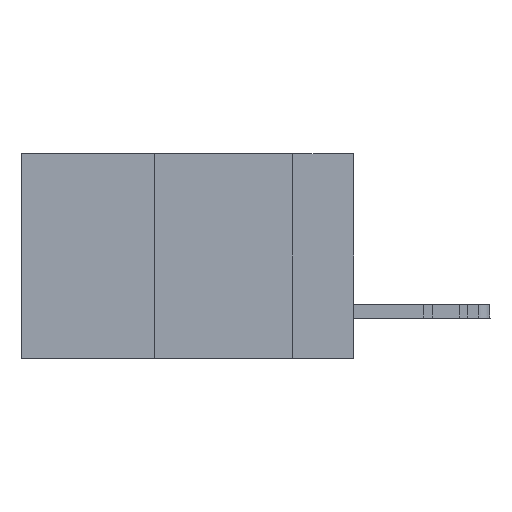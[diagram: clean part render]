
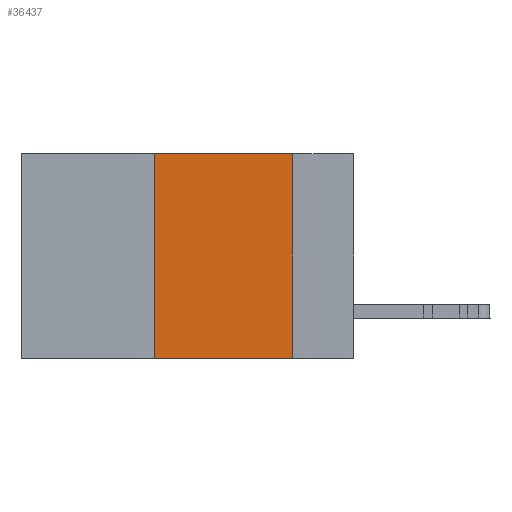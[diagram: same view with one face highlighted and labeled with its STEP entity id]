
A CAD part, left-side view. The second image highlights one B-rep face of the part: STEP entity #36437.
In plain terms, the highlighted planar face has unit normal (-1, 0, 0).
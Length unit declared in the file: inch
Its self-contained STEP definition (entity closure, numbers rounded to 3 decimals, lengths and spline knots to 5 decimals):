
#14 = LINE ( 'NONE', #45840, #43859 ) ;
#899 = ORIENTED_EDGE ( 'NONE', *, *, #42358, .F. ) ;
#2117 = DIRECTION ( 'NONE',  ( 0., 0., -1. ) ) ;
#2658 = VERTEX_POINT ( 'NONE', #26559 ) ;
#3344 = LINE ( 'NONE', #26875, #9012 ) ;
#9012 = VECTOR ( 'NONE', #49640, 39.37008 ) ;
#11147 = LINE ( 'NONE', #22791, #41113 ) ;
#11710 = ORIENTED_EDGE ( 'NONE', *, *, #39210, .F. ) ;
#12182 = DIRECTION ( 'NONE',  ( 0., 0., -1. ) ) ;
#12273 = VERTEX_POINT ( 'NONE', #48362 ) ;
#13768 = DIRECTION ( 'NONE',  ( 1., 0., 0. ) ) ;
#14005 = CARTESIAN_POINT ( 'NONE',  ( 0., 0.36, 0. ) ) ;
#16479 = CARTESIAN_POINT ( 'NONE',  ( 0., 0.11, -0.37 ) ) ;
#17064 = EDGE_CURVE ( 'NONE', #33422, #12273, #11147, .T. ) ;
#20358 = ORIENTED_EDGE ( 'NONE', *, *, #17064, .F. ) ;
#21111 = PLANE ( 'NONE',  #38744 ) ;
#22791 = CARTESIAN_POINT ( 'NONE',  ( 0., 0.6, 0. ) ) ;
#24957 = ORIENTED_EDGE ( 'NONE', *, *, #36163, .T. ) ;
#26559 = CARTESIAN_POINT ( 'NONE',  ( 0., 0.36, -0.37 ) ) ;
#26875 = CARTESIAN_POINT ( 'NONE',  ( 0., 0.36, 0. ) ) ;
#33422 = VERTEX_POINT ( 'NONE', #14005 ) ;
#34288 = CARTESIAN_POINT ( 'NONE',  ( 0., 0.6, -0.37 ) ) ;
#34822 = EDGE_LOOP ( 'NONE', ( #899, #20358, #11710, #24957 ) ) ;
#36163 = EDGE_CURVE ( 'NONE', #2658, #49295, #37347, .T. ) ;
#36437 = ADVANCED_FACE ( 'NONE', ( #39847 ), #21111, .F. ) ;
#37347 = LINE ( 'NONE', #34288, #45164 ) ;
#38230 = DIRECTION ( 'NONE',  ( 0., -1., 0. ) ) ;
#38744 = AXIS2_PLACEMENT_3D ( 'NONE', #40333, #13768, #2117 ) ;
#39210 = EDGE_CURVE ( 'NONE', #2658, #33422, #3344, .T. ) ;
#39847 = FACE_OUTER_BOUND ( 'NONE', #34822, .T. ) ;
#40333 = CARTESIAN_POINT ( 'NONE',  ( 0., 0.6, 0. ) ) ;
#41113 = VECTOR ( 'NONE', #38230, 39.37008 ) ;
#42358 = EDGE_CURVE ( 'NONE', #12273, #49295, #14, .T. ) ;
#43859 = VECTOR ( 'NONE', #12182, 39.37008 ) ;
#45164 = VECTOR ( 'NONE', #46178, 39.37008 ) ;
#45840 = CARTESIAN_POINT ( 'NONE',  ( 0., 0.11, 0. ) ) ;
#46178 = DIRECTION ( 'NONE',  ( 0., -1., 0. ) ) ;
#48362 = CARTESIAN_POINT ( 'NONE',  ( 0., 0.11, 0. ) ) ;
#49295 = VERTEX_POINT ( 'NONE', #16479 ) ;
#49640 = DIRECTION ( 'NONE',  ( 0., 0., 1. ) ) ;
